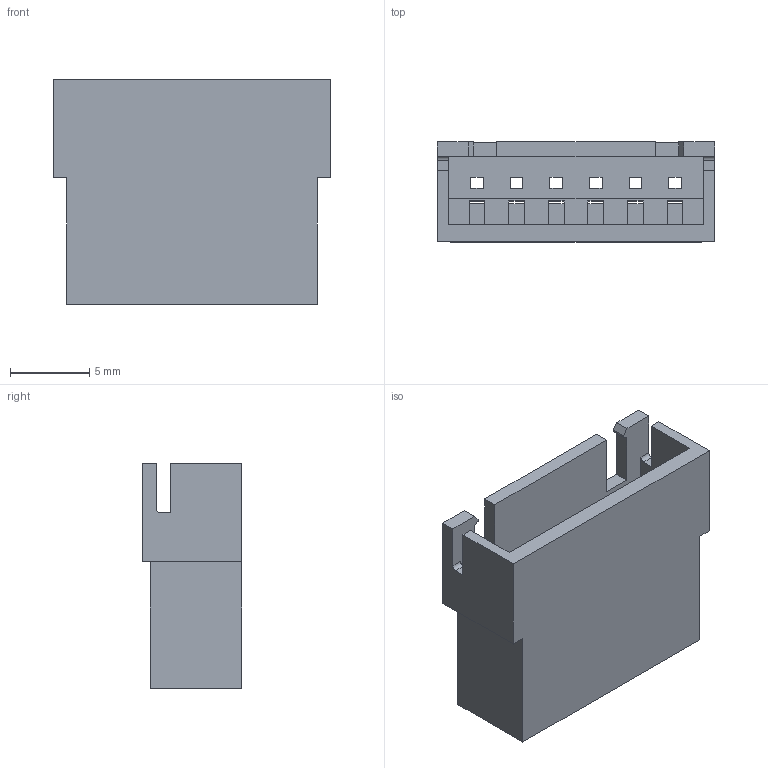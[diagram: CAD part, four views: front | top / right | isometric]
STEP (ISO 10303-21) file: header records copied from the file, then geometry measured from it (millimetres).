
FILE_DESCRIPTION (( 'STEP AP203' ), '1' );
FILE_NAME ('14K-506-210-AA1.STEP', '2024-02-23T14:31:51', ( '' ), ( '' ), 'SwSTEP 2.0', 'SolidWorks 2023', '' );
FILE_SCHEMA (( 'CONFIG_CONTROL_DESIGN' ));
Length unit declared in the file: millimetre
Products named in the file (1): 14K-506-210-AA1
Bounding box: 17.5 x 6.3 x 14.2 mm (x, y, z)
Volume: 744.4 mm3; surface area: 1709.5 mm2
Topology: 1 solids, 1 shells, 189 faces, 564 edges, 372 vertices
Faces by surface type: plane 185, cylinder 4
Entity records: 6335 total; most frequent: ORIENTED_EDGE 1128, CARTESIAN_POINT 1126, DIRECTION 952, EDGE_CURVE 564, VECTOR 556, LINE 556, VERTEX_POINT 372, EDGE_LOOP 208
